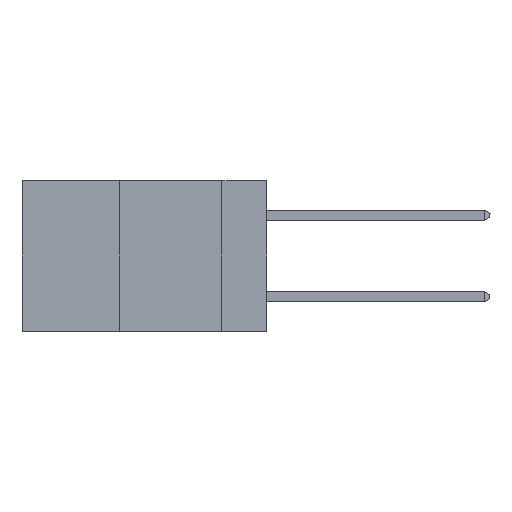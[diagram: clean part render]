
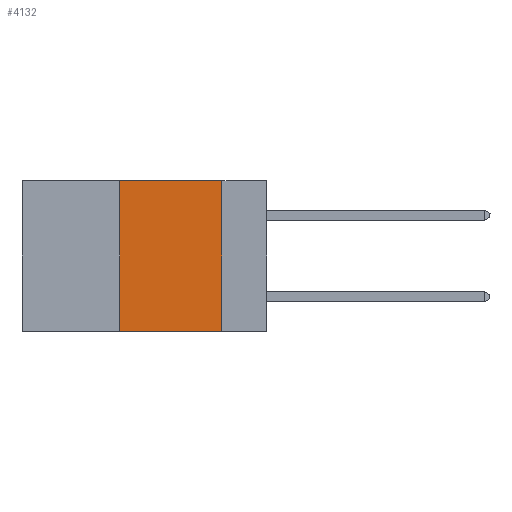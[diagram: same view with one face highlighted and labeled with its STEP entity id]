
A CAD part, left-side view. The second image highlights one B-rep face of the part: STEP entity #4132.
In plain terms, the highlighted planar face has unit normal (-1, 0, 0).
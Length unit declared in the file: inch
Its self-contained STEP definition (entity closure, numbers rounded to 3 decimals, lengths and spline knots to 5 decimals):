
#157 = EDGE_CURVE ( 'NONE', #5870, #10895, #3075, .T. ) ;
#531 = DIRECTION ( 'NONE',  ( 1., 0., 0. ) ) ;
#1489 = VECTOR ( 'NONE', #9885, 39.37008 ) ;
#1852 = VECTOR ( 'NONE', #10079, 39.37008 ) ;
#2061 = EDGE_LOOP ( 'NONE', ( #5136, #11601, #8619, #4130 ) ) ;
#2514 = DIRECTION ( 'NONE',  ( 0., -1., 0. ) ) ;
#2570 = EDGE_CURVE ( 'NONE', #4889, #10895, #5830, .T. ) ;
#2744 = EDGE_CURVE ( 'NONE', #5870, #5749, #10018, .T. ) ;
#3065 = CARTESIAN_POINT ( 'NONE',  ( 0., 0.6, 0. ) ) ;
#3075 = LINE ( 'NONE', #9939, #1489 ) ;
#3509 = EDGE_CURVE ( 'NONE', #5749, #4889, #6887, .T. ) ;
#3581 = CARTESIAN_POINT ( 'NONE',  ( 0., 0.36, -0.37 ) ) ;
#4037 = DIRECTION ( 'NONE',  ( 0., 0., -1. ) ) ;
#4130 = ORIENTED_EDGE ( 'NONE', *, *, #157, .T. ) ;
#4132 = ADVANCED_FACE ( 'NONE', ( #5471 ), #12549, .F. ) ;
#4889 = VERTEX_POINT ( 'NONE', #10045 ) ;
#5136 = ORIENTED_EDGE ( 'NONE', *, *, #2570, .F. ) ;
#5297 = CARTESIAN_POINT ( 'NONE',  ( 0., 0.11, -0.37 ) ) ;
#5471 = FACE_OUTER_BOUND ( 'NONE', #2061, .T. ) ;
#5749 = VERTEX_POINT ( 'NONE', #8375 ) ;
#5830 = LINE ( 'NONE', #7641, #10336 ) ;
#5870 = VERTEX_POINT ( 'NONE', #3581 ) ;
#6600 = CARTESIAN_POINT ( 'NONE',  ( 0., 0.6, 0. ) ) ;
#6887 = LINE ( 'NONE', #3065, #10945 ) ;
#7641 = CARTESIAN_POINT ( 'NONE',  ( 0., 0.11, 0. ) ) ;
#8375 = CARTESIAN_POINT ( 'NONE',  ( 0., 0.36, 0. ) ) ;
#8589 = DIRECTION ( 'NONE',  ( 0., 0., -1. ) ) ;
#8619 = ORIENTED_EDGE ( 'NONE', *, *, #2744, .F. ) ;
#8718 = AXIS2_PLACEMENT_3D ( 'NONE', #6600, #531, #8589 ) ;
#9079 = CARTESIAN_POINT ( 'NONE',  ( 0., 0.36, 0. ) ) ;
#9885 = DIRECTION ( 'NONE',  ( 0., -1., 0. ) ) ;
#9939 = CARTESIAN_POINT ( 'NONE',  ( 0., 0.6, -0.37 ) ) ;
#10018 = LINE ( 'NONE', #9079, #1852 ) ;
#10045 = CARTESIAN_POINT ( 'NONE',  ( 0., 0.11, 0. ) ) ;
#10079 = DIRECTION ( 'NONE',  ( 0., 0., 1. ) ) ;
#10336 = VECTOR ( 'NONE', #4037, 39.37008 ) ;
#10895 = VERTEX_POINT ( 'NONE', #5297 ) ;
#10945 = VECTOR ( 'NONE', #2514, 39.37008 ) ;
#11601 = ORIENTED_EDGE ( 'NONE', *, *, #3509, .F. ) ;
#12549 = PLANE ( 'NONE',  #8718 ) ;
